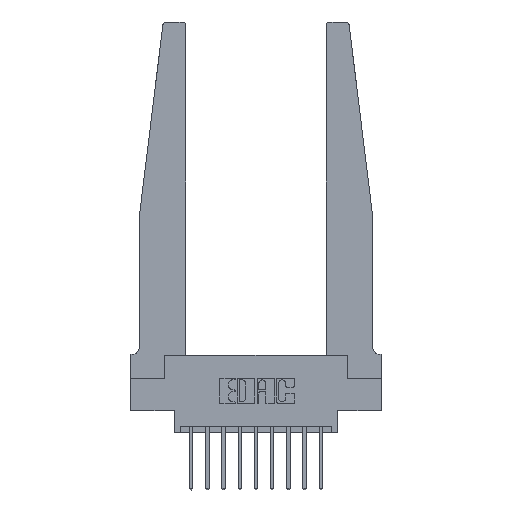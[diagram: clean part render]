
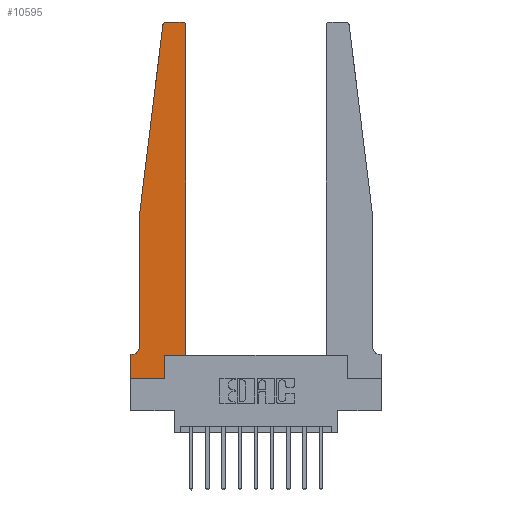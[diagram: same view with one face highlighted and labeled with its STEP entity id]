
A CAD part, top view. The second image highlights one B-rep face of the part: STEP entity #10595.
In plain terms, the highlighted planar face has unit normal (0, 0, 1).
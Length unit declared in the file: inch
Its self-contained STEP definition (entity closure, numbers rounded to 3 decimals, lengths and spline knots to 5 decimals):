
#119 = CARTESIAN_POINT ( 'NONE',  ( 0., 0.1875, 0.37 ) ) ;
#268 = EDGE_CURVE ( 'NONE', #14791, #11148, #13455, .T. ) ;
#273 = ORIENTED_EDGE ( 'NONE', *, *, #1797, .T. ) ;
#377 = VERTEX_POINT ( 'NONE', #15070 ) ;
#389 = DIRECTION ( 'NONE',  ( 0., -1., 0. ) ) ;
#393 = CARTESIAN_POINT ( 'NONE',  ( 0.065, 0.2375, 0.37 ) ) ;
#420 = LINE ( 'NONE', #10994, #3206 ) ;
#636 = EDGE_LOOP ( 'NONE', ( #3055, #273, #5814, #8994, #1937, #11746, #10279, #1190, #6905, #1000, #10869, #13564 ) ) ;
#766 = AXIS2_PLACEMENT_3D ( 'NONE', #14902, #7883, #800 ) ;
#800 = DIRECTION ( 'NONE',  ( 1., 0., 0. ) ) ;
#834 = CIRCLE ( 'NONE', #14511, 0.05 ) ;
#1000 = ORIENTED_EDGE ( 'NONE', *, *, #12144, .T. ) ;
#1190 = ORIENTED_EDGE ( 'NONE', *, *, #6529, .T. ) ;
#1224 = FACE_OUTER_BOUND ( 'NONE', #636, .T. ) ;
#1513 = DIRECTION ( 'NONE',  ( 0., -1., 0. ) ) ;
#1703 = VERTEX_POINT ( 'NONE', #2943 ) ;
#1797 = EDGE_CURVE ( 'NONE', #6370, #9968, #4388, .T. ) ;
#1882 = DIRECTION ( 'NONE',  ( 1., 0., 0. ) ) ;
#1937 = ORIENTED_EDGE ( 'NONE', *, *, #11116, .T. ) ;
#2122 = DIRECTION ( 'NONE',  ( 0., 0., 1. ) ) ;
#2266 = CARTESIAN_POINT ( 'NONE',  ( 0.425, 0.18, 0.37 ) ) ;
#2526 = DIRECTION ( 'NONE',  ( 0., 1., 0. ) ) ;
#2794 = CARTESIAN_POINT ( 'NONE',  ( 0.065, 1.25, 0.37 ) ) ;
#2943 = CARTESIAN_POINT ( 'NONE',  ( 0.2605, 0., 0.37 ) ) ;
#2991 = DIRECTION ( 'NONE',  ( 1., 0., 0. ) ) ;
#3055 = ORIENTED_EDGE ( 'NONE', *, *, #3352, .T. ) ;
#3206 = VECTOR ( 'NONE', #1513, 39.37008 ) ;
#3352 = EDGE_CURVE ( 'NONE', #8825, #6370, #12644, .T. ) ;
#3513 = DIRECTION ( 'NONE',  ( 0., 1., 0. ) ) ;
#3555 = VERTEX_POINT ( 'NONE', #2266 ) ;
#3863 = CARTESIAN_POINT ( 'NONE',  ( 0.395, 2.75, 0.37 ) ) ;
#4008 = VERTEX_POINT ( 'NONE', #6105 ) ;
#4177 = EDGE_CURVE ( 'NONE', #9968, #10103, #5791, .T. ) ;
#4284 = CARTESIAN_POINT ( 'NONE',  ( 0.065, 1.25, 0.37 ) ) ;
#4388 = CIRCLE ( 'NONE', #766, 0.03 ) ;
#4491 = VERTEX_POINT ( 'NONE', #10770 ) ;
#4849 = CARTESIAN_POINT ( 'NONE',  ( 0.065, 1.25, 0.37 ) ) ;
#4937 = DIRECTION ( 'NONE',  ( 1., 0., 0. ) ) ;
#5357 = CARTESIAN_POINT ( 'NONE',  ( 0., 0., 0.37 ) ) ;
#5425 = VECTOR ( 'NONE', #11375, 39.37008 ) ;
#5791 = LINE ( 'NONE', #4284, #5425 ) ;
#5814 = ORIENTED_EDGE ( 'NONE', *, *, #4177, .T. ) ;
#5893 = VECTOR ( 'NONE', #3513, 39.37008 ) ;
#5977 = CARTESIAN_POINT ( 'NONE',  ( 0.015, 0.1875, 0.37 ) ) ;
#5990 = DIRECTION ( 'NONE',  ( 0., 0., -1. ) ) ;
#6044 = CARTESIAN_POINT ( 'NONE',  ( 0., 0.1875, 0.37 ) ) ;
#6105 = CARTESIAN_POINT ( 'NONE',  ( 0., 0., 0.37 ) ) ;
#6370 = VERTEX_POINT ( 'NONE', #10816 ) ;
#6384 = CARTESIAN_POINT ( 'NONE',  ( 0.065, 0.1875, 0.37 ) ) ;
#6529 = EDGE_CURVE ( 'NONE', #4008, #1703, #10212, .T. ) ;
#6905 = ORIENTED_EDGE ( 'NONE', *, *, #13471, .T. ) ;
#7031 = VECTOR ( 'NONE', #2991, 39.37008 ) ;
#7521 = AXIS2_PLACEMENT_3D ( 'NONE', #9225, #2122, #10408 ) ;
#7757 = CARTESIAN_POINT ( 'NONE',  ( 0.425, 0.18, 0.37 ) ) ;
#7775 = CARTESIAN_POINT ( 'NONE',  ( 0.25, 2.75, 0.37 ) ) ;
#7883 = DIRECTION ( 'NONE',  ( 0., 0., 1. ) ) ;
#8545 = AXIS2_PLACEMENT_3D ( 'NONE', #119, #12015, #4937 ) ;
#8804 = VECTOR ( 'NONE', #2526, 39.37008 ) ;
#8825 = VERTEX_POINT ( 'NONE', #3863 ) ;
#8994 = ORIENTED_EDGE ( 'NONE', *, *, #13652, .T. ) ;
#9080 = LINE ( 'NONE', #14053, #5893 ) ;
#9225 = CARTESIAN_POINT ( 'NONE',  ( 0.395, 2.72, 0.37 ) ) ;
#9539 = VECTOR ( 'NONE', #1882, 39.37008 ) ;
#9559 = VECTOR ( 'NONE', #13688, 39.37008 ) ;
#9636 = VECTOR ( 'NONE', #389, 39.37008 ) ;
#9643 = CARTESIAN_POINT ( 'NONE',  ( 0.425, 0.18, 0.37 ) ) ;
#9802 = CIRCLE ( 'NONE', #7521, 0.03 ) ;
#9921 = EDGE_CURVE ( 'NONE', #377, #8825, #9802, .T. ) ;
#9968 = VERTEX_POINT ( 'NONE', #15107 ) ;
#9986 = LINE ( 'NONE', #2794, #9636 ) ;
#10103 = VERTEX_POINT ( 'NONE', #4849 ) ;
#10156 = VERTEX_POINT ( 'NONE', #393 ) ;
#10212 = LINE ( 'NONE', #5357, #7031 ) ;
#10279 = ORIENTED_EDGE ( 'NONE', *, *, #12593, .T. ) ;
#10376 = VECTOR ( 'NONE', #13525, 39.37008 ) ;
#10408 = DIRECTION ( 'NONE',  ( 1., 0., 0. ) ) ;
#10595 = ADVANCED_FACE ( 'NONE', ( #1224 ), #14286, .T. ) ;
#10770 = CARTESIAN_POINT ( 'NONE',  ( 0.2605, 0.18, 0.37 ) ) ;
#10816 = CARTESIAN_POINT ( 'NONE',  ( 0.27653, 2.75, 0.37 ) ) ;
#10869 = ORIENTED_EDGE ( 'NONE', *, *, #11740, .T. ) ;
#10994 = CARTESIAN_POINT ( 'NONE',  ( 0., 0., 0.37 ) ) ;
#11116 = EDGE_CURVE ( 'NONE', #10156, #14791, #834, .T. ) ;
#11148 = VERTEX_POINT ( 'NONE', #6044 ) ;
#11194 = LINE ( 'NONE', #9643, #8804 ) ;
#11375 = DIRECTION ( 'NONE',  ( -0.122, -0.992, 0. ) ) ;
#11740 = EDGE_CURVE ( 'NONE', #3555, #377, #11194, .T. ) ;
#11746 = ORIENTED_EDGE ( 'NONE', *, *, #268, .T. ) ;
#12015 = DIRECTION ( 'NONE',  ( 0., 0., 1. ) ) ;
#12144 = EDGE_CURVE ( 'NONE', #4491, #3555, #12994, .T. ) ;
#12593 = EDGE_CURVE ( 'NONE', #11148, #4008, #420, .T. ) ;
#12644 = LINE ( 'NONE', #7775, #9559 ) ;
#12994 = LINE ( 'NONE', #7757, #9539 ) ;
#13059 = CARTESIAN_POINT ( 'NONE',  ( 0.015, 0.2375, 0.37 ) ) ;
#13455 = LINE ( 'NONE', #6384, #10376 ) ;
#13471 = EDGE_CURVE ( 'NONE', #1703, #4491, #9080, .T. ) ;
#13525 = DIRECTION ( 'NONE',  ( -1., 0., 0. ) ) ;
#13564 = ORIENTED_EDGE ( 'NONE', *, *, #9921, .T. ) ;
#13652 = EDGE_CURVE ( 'NONE', #10103, #10156, #9986, .T. ) ;
#13688 = DIRECTION ( 'NONE',  ( -1., 0., 0. ) ) ;
#14053 = CARTESIAN_POINT ( 'NONE',  ( 0.2605, 0.18, 0.37 ) ) ;
#14220 = DIRECTION ( 'NONE',  ( -1., 0., 0. ) ) ;
#14286 = PLANE ( 'NONE',  #8545 ) ;
#14511 = AXIS2_PLACEMENT_3D ( 'NONE', #13059, #5990, #14220 ) ;
#14791 = VERTEX_POINT ( 'NONE', #5977 ) ;
#14902 = CARTESIAN_POINT ( 'NONE',  ( 0.27653, 2.72, 0.37 ) ) ;
#15070 = CARTESIAN_POINT ( 'NONE',  ( 0.425, 2.72, 0.37 ) ) ;
#15107 = CARTESIAN_POINT ( 'NONE',  ( 0.24675, 2.72367, 0.37 ) ) ;
